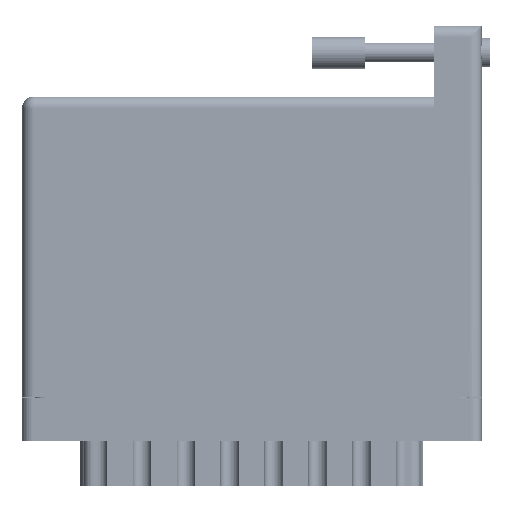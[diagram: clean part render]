
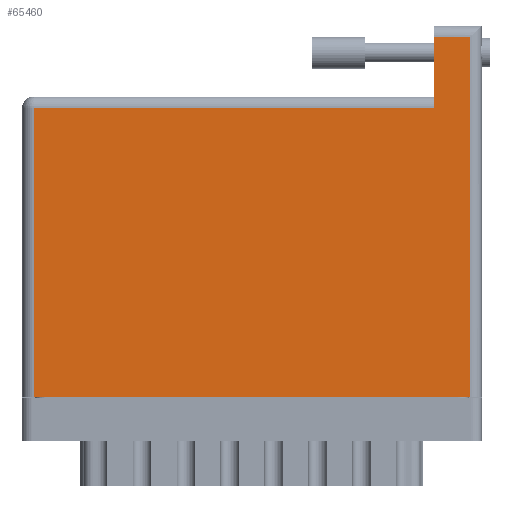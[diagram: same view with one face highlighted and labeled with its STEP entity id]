
A CAD part, front view. The second image highlights one B-rep face of the part: STEP entity #65460.
In plain terms, the highlighted face is planar.
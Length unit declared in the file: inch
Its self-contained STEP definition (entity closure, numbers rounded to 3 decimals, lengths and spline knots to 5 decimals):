
#1455 = CARTESIAN_POINT ( 'NONE',  ( 0., 1.705, 0. ) ) ;
#2421 = CARTESIAN_POINT ( 'NONE',  ( 0.07, 0., 0. ) ) ;
#6983 = EDGE_LOOP ( 'NONE', ( #35885, #50644, #23671, #57859, #59913, #24001 ) ) ;
#8335 = CARTESIAN_POINT ( 'NONE',  ( 2.438, 2.125, 0. ) ) ;
#9343 = LINE ( 'NONE', #17691, #32351 ) ;
#10344 = CARTESIAN_POINT ( 'NONE',  ( 2.648, 2.125, 0. ) ) ;
#10999 = LINE ( 'NONE', #2421, #28509 ) ;
#12006 = EDGE_CURVE ( 'NONE', #59815, #39748, #65418, .T. ) ;
#12374 = CARTESIAN_POINT ( 'NONE',  ( 2.648, 2.195, 0. ) ) ;
#16835 = EDGE_CURVE ( 'NONE', #39748, #71907, #9343, .T. ) ;
#17691 = CARTESIAN_POINT ( 'NONE',  ( 2.438, 2.195, 0. ) ) ;
#20519 = LINE ( 'NONE', #12374, #30624 ) ;
#21192 = VERTEX_POINT ( 'NONE', #41485 ) ;
#22976 = AXIS2_PLACEMENT_3D ( 'NONE', #48054, #54753, #66314 ) ;
#23036 = EDGE_CURVE ( 'NONE', #43470, #21192, #10999, .T. ) ;
#23671 = ORIENTED_EDGE ( 'NONE', *, *, #49945, .T. ) ;
#24001 = ORIENTED_EDGE ( 'NONE', *, *, #16835, .T. ) ;
#28509 = VECTOR ( 'NONE', #60551, 39.37008 ) ;
#29021 = DIRECTION ( 'NONE',  ( 0., -1., 0. ) ) ;
#29606 = DIRECTION ( 'NONE',  ( 0., 1., 0. ) ) ;
#30624 = VECTOR ( 'NONE', #29606, 39.37008 ) ;
#31648 = CARTESIAN_POINT ( 'NONE',  ( 2.438, 1.705, 0. ) ) ;
#32351 = VECTOR ( 'NONE', #29021, 39.37008 ) ;
#35417 = CARTESIAN_POINT ( 'NONE',  ( 0., 0., 0. ) ) ;
#35542 = CARTESIAN_POINT ( 'NONE',  ( 2.648, 0., 0. ) ) ;
#35885 = ORIENTED_EDGE ( 'NONE', *, *, #70463, .T. ) ;
#39357 = LINE ( 'NONE', #35417, #48568 ) ;
#39748 = VERTEX_POINT ( 'NONE', #8335 ) ;
#41485 = CARTESIAN_POINT ( 'NONE',  ( 0.07, 0., 0. ) ) ;
#43470 = VERTEX_POINT ( 'NONE', #62145 ) ;
#48054 = CARTESIAN_POINT ( 'NONE',  ( 0., 1.775, 0. ) ) ;
#48568 = VECTOR ( 'NONE', #70959, 39.37008 ) ;
#49945 = EDGE_CURVE ( 'NONE', #21192, #66521, #39357, .T. ) ;
#50644 = ORIENTED_EDGE ( 'NONE', *, *, #23036, .T. ) ;
#52233 = CARTESIAN_POINT ( 'NONE',  ( 0., 2.125, 0. ) ) ;
#53276 = EDGE_CURVE ( 'NONE', #66521, #59815, #20519, .T. ) ;
#54753 = DIRECTION ( 'NONE',  ( 0., 0., -1. ) ) ;
#56262 = VECTOR ( 'NONE', #70542, 39.37008 ) ;
#56379 = VECTOR ( 'NONE', #61148, 39.37008 ) ;
#57859 = ORIENTED_EDGE ( 'NONE', *, *, #53276, .T. ) ;
#59815 = VERTEX_POINT ( 'NONE', #10344 ) ;
#59913 = ORIENTED_EDGE ( 'NONE', *, *, #12006, .T. ) ;
#60385 = PLANE ( 'NONE',  #22976 ) ;
#60551 = DIRECTION ( 'NONE',  ( 0., -1., 0. ) ) ;
#61148 = DIRECTION ( 'NONE',  ( -1., 0., 0. ) ) ;
#62145 = CARTESIAN_POINT ( 'NONE',  ( 0.07, 1.705, 0. ) ) ;
#65418 = LINE ( 'NONE', #52233, #56262 ) ;
#65460 = ADVANCED_FACE ( 'NONE', ( #73622 ), #60385, .F. ) ;
#66314 = DIRECTION ( 'NONE',  ( -1., 0., 0. ) ) ;
#66521 = VERTEX_POINT ( 'NONE', #35542 ) ;
#70463 = EDGE_CURVE ( 'NONE', #71907, #43470, #71171, .T. ) ;
#70542 = DIRECTION ( 'NONE',  ( -1., 0., 0. ) ) ;
#70959 = DIRECTION ( 'NONE',  ( 1., 0., 0. ) ) ;
#71171 = LINE ( 'NONE', #1455, #56379 ) ;
#71907 = VERTEX_POINT ( 'NONE', #31648 ) ;
#73622 = FACE_OUTER_BOUND ( 'NONE', #6983, .T. ) ;
